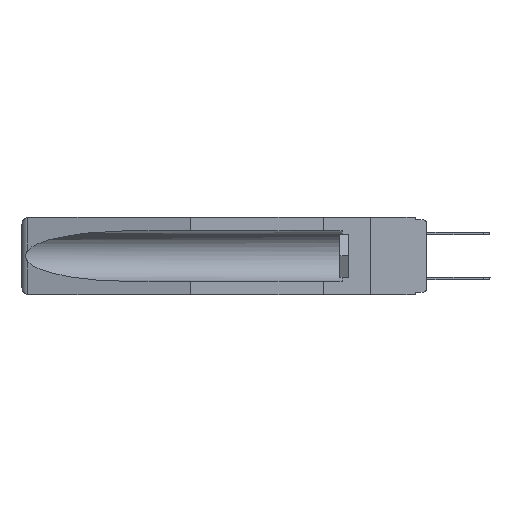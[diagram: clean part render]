
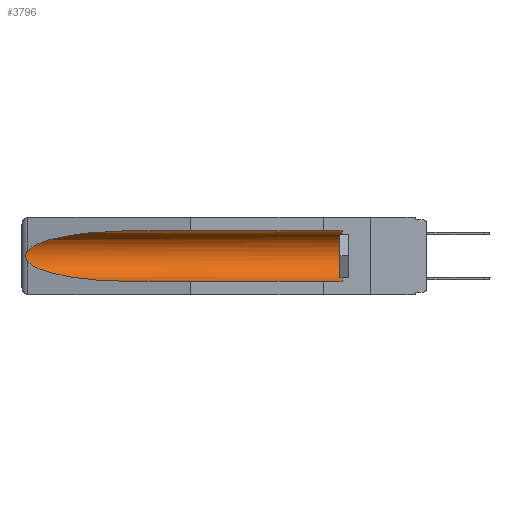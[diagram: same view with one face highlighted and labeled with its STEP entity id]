
A CAD part, left-side view. The second image highlights one B-rep face of the part: STEP entity #3796.
In plain terms, the highlighted cylindrical face has radius 2.857 mm (diameter 5.715 mm), a partial arc.
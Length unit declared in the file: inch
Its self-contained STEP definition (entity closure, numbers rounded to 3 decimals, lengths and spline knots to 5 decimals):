
#414 = VERTEX_POINT ( 'NONE', #14005 ) ;
#1098 = CARTESIAN_POINT ( 'NONE',  ( 0.25451, 1.48313, -0.24835 ) ) ;
#1112 = VERTEX_POINT ( 'NONE', #2324 ) ;
#1136 = VECTOR ( 'NONE', #13315, 39.37008 ) ;
#1213 = CARTESIAN_POINT ( 'NONE',  ( 0.2675, 1.53308, -0.17534 ) ) ;
#1253 = CARTESIAN_POINT ( 'NONE',  ( 0.21114, 1.30732, -0.284 ) ) ;
#1379 = B_SPLINE_CURVE_WITH_KNOTS ( 'NONE', 3,
 ( #21195, #21049, #21274, #4843, #6138, #1213, #2970, #14437, #17681, #14360 ),
 .UNSPECIFIED., .F., .F.,
 ( 4, 2, 2, 2, 4 ),
 ( 0., 0.00029, 0.00058, 0.00087, 0.00117 ),
 .UNSPECIFIED. ) ;
#1515 = CARTESIAN_POINT ( 'NONE',  ( 0.26537, 1.52718, -0.14972 ) ) ;
#1653 =( BOUNDED_CURVE ( )  B_SPLINE_CURVE ( 3, ( #9465, #1098, #1253, #2934 ),
 .UNSPECIFIED., .F., .F. ) 
 B_SPLINE_CURVE_WITH_KNOTS ( ( 4, 4 ),
 ( 0.1948, 1.5708 ),
 .UNSPECIFIED. ) 
 CURVE ( )  GEOMETRIC_REPRESENTATION_ITEM ( )  RATIONAL_B_SPLINE_CURVE ( ( 1., 0.848, 0.848, 1. ) ) 
 REPRESENTATION_ITEM ( '' )  );
#1726 = ORIENTED_EDGE ( 'NONE', *, *, #16185, .T. ) ;
#2085 = CARTESIAN_POINT ( 'NONE',  ( 0.155, 0.126, -0.1715 ) ) ;
#2324 = CARTESIAN_POINT ( 'NONE',  ( 0.26537, 1.52718, -0.14972 ) ) ;
#2351 = CARTESIAN_POINT ( 'NONE',  ( 0.155, -0.30754, -0.1715 ) ) ;
#2548 = EDGE_CURVE ( 'NONE', #3001, #3560, #4074, .T. ) ;
#2704 = LINE ( 'NONE', #19952, #1136 ) ;
#2934 = CARTESIAN_POINT ( 'NONE',  ( 0.155, 1.07973, -0.284 ) ) ;
#2970 = CARTESIAN_POINT ( 'NONE',  ( 0.2673, 1.53269, -0.17917 ) ) ;
#3001 = VERTEX_POINT ( 'NONE', #21017 ) ;
#3560 = VERTEX_POINT ( 'NONE', #6562 ) ;
#3796 = ADVANCED_FACE ( 'NONE', ( #11232 ), #15083, .F. ) ;
#3847 = ORIENTED_EDGE ( 'NONE', *, *, #14087, .F. ) ;
#4074 = CIRCLE ( 'NONE', #4129, 0.1125 ) ;
#4129 = AXIS2_PLACEMENT_3D ( 'NONE', #2085, #11729, #13585 ) ;
#4179 = ORIENTED_EDGE ( 'NONE', *, *, #8367, .T. ) ;
#4843 = CARTESIAN_POINT ( 'NONE',  ( 0.2673, 1.5327, -0.16383 ) ) ;
#6138 = CARTESIAN_POINT ( 'NONE',  ( 0.2675, 1.53308, -0.16763 ) ) ;
#6562 = CARTESIAN_POINT ( 'NONE',  ( 0.155, 0.126, -0.059 ) ) ;
#7645 = VECTOR ( 'NONE', #16047, 39.37008 ) ;
#7690 = CARTESIAN_POINT ( 'NONE',  ( 0.155, -0.30754, -0.284 ) ) ;
#7957 = ORIENTED_EDGE ( 'NONE', *, *, #8172, .T. ) ;
#8172 = EDGE_CURVE ( 'NONE', #12602, #1112, #13132, .T. ) ;
#8367 = EDGE_CURVE ( 'NONE', #414, #13115, #1653, .T. ) ;
#9465 = CARTESIAN_POINT ( 'NONE',  ( 0.26537, 1.52718, -0.19328 ) ) ;
#9572 = CARTESIAN_POINT ( 'NONE',  ( 0.25451, 1.48313, -0.09465 ) ) ;
#9723 = EDGE_LOOP ( 'NONE', ( #7957, #17609, #4179, #3847, #17419, #1726 ) ) ;
#10469 = LINE ( 'NONE', #7690, #7645 ) ;
#11232 = FACE_OUTER_BOUND ( 'NONE', #9723, .T. ) ;
#11370 = CARTESIAN_POINT ( 'NONE',  ( 0.21114, 1.30732, -0.059 ) ) ;
#11729 = DIRECTION ( 'NONE',  ( 0., -1., 0. ) ) ;
#12120 = CARTESIAN_POINT ( 'NONE',  ( 0.155, 1.07973, -0.059 ) ) ;
#12602 = VERTEX_POINT ( 'NONE', #12120 ) ;
#13115 = VERTEX_POINT ( 'NONE', #18482 ) ;
#13132 =( BOUNDED_CURVE ( )  B_SPLINE_CURVE ( 3, ( #17819, #11370, #9572, #1515 ),
 .UNSPECIFIED., .F., .T. ) 
 B_SPLINE_CURVE_WITH_KNOTS ( ( 4, 4 ),
 ( 4.71239, 6.08839 ),
 .UNSPECIFIED. ) 
 CURVE ( )  GEOMETRIC_REPRESENTATION_ITEM ( )  RATIONAL_B_SPLINE_CURVE ( ( 1., 0.848, 0.848, 1. ) ) 
 REPRESENTATION_ITEM ( '' )  );
#13315 = DIRECTION ( 'NONE',  ( 0., 1., 0. ) ) ;
#13585 = DIRECTION ( 'NONE',  ( 0., 0., 1. ) ) ;
#14005 = CARTESIAN_POINT ( 'NONE',  ( 0.26537, 1.52718, -0.19328 ) ) ;
#14087 = EDGE_CURVE ( 'NONE', #3001, #13115, #10469, .T. ) ;
#14186 = AXIS2_PLACEMENT_3D ( 'NONE', #2351, #17337, #19058 ) ;
#14360 = CARTESIAN_POINT ( 'NONE',  ( 0.26537, 1.52718, -0.19328 ) ) ;
#14437 = CARTESIAN_POINT ( 'NONE',  ( 0.26655, 1.53094, -0.18657 ) ) ;
#15083 = CYLINDRICAL_SURFACE ( 'NONE', #14186, 0.1125 ) ;
#16047 = DIRECTION ( 'NONE',  ( 0., 1., 0. ) ) ;
#16052 = EDGE_CURVE ( 'NONE', #1112, #414, #1379, .T. ) ;
#16185 = EDGE_CURVE ( 'NONE', #3560, #12602, #2704, .T. ) ;
#17337 = DIRECTION ( 'NONE',  ( 0., 1., 0. ) ) ;
#17419 = ORIENTED_EDGE ( 'NONE', *, *, #2548, .T. ) ;
#17609 = ORIENTED_EDGE ( 'NONE', *, *, #16052, .T. ) ;
#17681 = CARTESIAN_POINT ( 'NONE',  ( 0.26597, 1.5296, -0.19026 ) ) ;
#17819 = CARTESIAN_POINT ( 'NONE',  ( 0.155, 1.07973, -0.059 ) ) ;
#18482 = CARTESIAN_POINT ( 'NONE',  ( 0.155, 1.07973, -0.284 ) ) ;
#19058 = DIRECTION ( 'NONE',  ( 0., 0., 1. ) ) ;
#19952 = CARTESIAN_POINT ( 'NONE',  ( 0.155, -0.30754, -0.059 ) ) ;
#21017 = CARTESIAN_POINT ( 'NONE',  ( 0.155, 0.126, -0.284 ) ) ;
#21049 = CARTESIAN_POINT ( 'NONE',  ( 0.26597, 1.52961, -0.15275 ) ) ;
#21195 = CARTESIAN_POINT ( 'NONE',  ( 0.26537, 1.52718, -0.14972 ) ) ;
#21274 = CARTESIAN_POINT ( 'NONE',  ( 0.26654, 1.53092, -0.15636 ) ) ;
